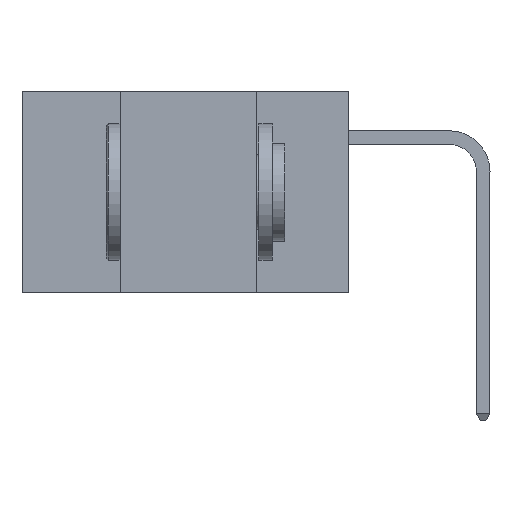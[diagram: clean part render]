
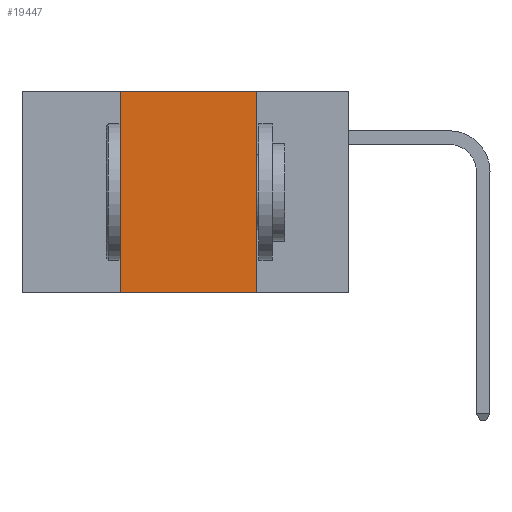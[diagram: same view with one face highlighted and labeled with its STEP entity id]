
A CAD part, left-side view. The second image highlights one B-rep face of the part: STEP entity #19447.
In plain terms, the highlighted planar face has unit normal (-1, 0, 0).
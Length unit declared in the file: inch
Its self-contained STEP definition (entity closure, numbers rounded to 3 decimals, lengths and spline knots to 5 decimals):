
#1577 = VECTOR ( 'NONE', #1628, 39.37008 ) ;
#1628 = DIRECTION ( 'NONE',  ( 0., 0., -1. ) ) ;
#1636 = VECTOR ( 'NONE', #15170, 39.37008 ) ;
#2386 = CARTESIAN_POINT ( 'NONE',  ( 0., 0.6, -0.37 ) ) ;
#2529 = CARTESIAN_POINT ( 'NONE',  ( 0., 0.42, -0.37 ) ) ;
#3111 = EDGE_CURVE ( 'NONE', #17853, #30184, #6471, .T. ) ;
#3982 = LINE ( 'NONE', #2386, #22799 ) ;
#4674 = LINE ( 'NONE', #6773, #1577 ) ;
#5063 = ORIENTED_EDGE ( 'NONE', *, *, #9034, .F. ) ;
#5615 = DIRECTION ( 'NONE',  ( 0., -1., 0. ) ) ;
#6471 = LINE ( 'NONE', #10220, #22256 ) ;
#6592 = EDGE_CURVE ( 'NONE', #31493, #16735, #3982, .T. ) ;
#6773 = CARTESIAN_POINT ( 'NONE',  ( 0., 0.17, 0. ) ) ;
#7413 = DIRECTION ( 'NONE',  ( 0., -1., 0. ) ) ;
#9034 = EDGE_CURVE ( 'NONE', #31493, #17853, #28581, .T. ) ;
#10134 = DIRECTION ( 'NONE',  ( 1., 0., 0. ) ) ;
#10220 = CARTESIAN_POINT ( 'NONE',  ( 0., 0.6, 0. ) ) ;
#10453 = CARTESIAN_POINT ( 'NONE',  ( 0., 0.17, 0. ) ) ;
#11362 = ORIENTED_EDGE ( 'NONE', *, *, #20939, .F. ) ;
#12181 = ORIENTED_EDGE ( 'NONE', *, *, #6592, .T. ) ;
#13032 = CARTESIAN_POINT ( 'NONE',  ( 0., 0.6, 0. ) ) ;
#13756 = ORIENTED_EDGE ( 'NONE', *, *, #3111, .F. ) ;
#15170 = DIRECTION ( 'NONE',  ( 0., 0., 1. ) ) ;
#15526 = DIRECTION ( 'NONE',  ( 0., 0., -1. ) ) ;
#16297 = FACE_OUTER_BOUND ( 'NONE', #21186, .T. ) ;
#16735 = VERTEX_POINT ( 'NONE', #21914 ) ;
#17853 = VERTEX_POINT ( 'NONE', #28931 ) ;
#19447 = ADVANCED_FACE ( 'NONE', ( #16297 ), #20355, .F. ) ;
#20355 = PLANE ( 'NONE',  #21733 ) ;
#20939 = EDGE_CURVE ( 'NONE', #30184, #16735, #4674, .T. ) ;
#21186 = EDGE_LOOP ( 'NONE', ( #11362, #13756, #5063, #12181 ) ) ;
#21733 = AXIS2_PLACEMENT_3D ( 'NONE', #13032, #10134, #15526 ) ;
#21914 = CARTESIAN_POINT ( 'NONE',  ( 0., 0.17, -0.37 ) ) ;
#22256 = VECTOR ( 'NONE', #5615, 39.37008 ) ;
#22799 = VECTOR ( 'NONE', #7413, 39.37008 ) ;
#25253 = CARTESIAN_POINT ( 'NONE',  ( 0., 0.42, 0. ) ) ;
#28581 = LINE ( 'NONE', #25253, #1636 ) ;
#28931 = CARTESIAN_POINT ( 'NONE',  ( 0., 0.42, 0. ) ) ;
#30184 = VERTEX_POINT ( 'NONE', #10453 ) ;
#31493 = VERTEX_POINT ( 'NONE', #2529 ) ;
